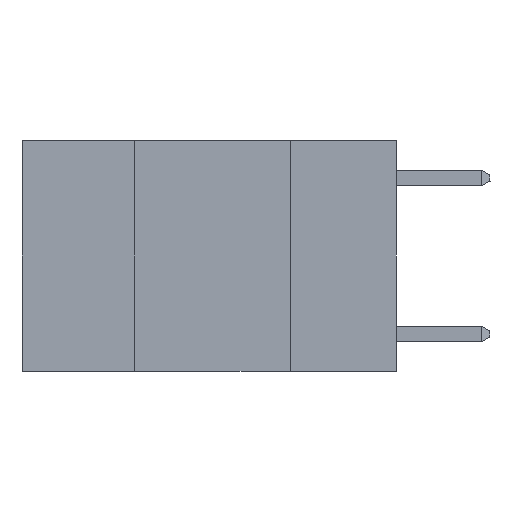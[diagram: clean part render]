
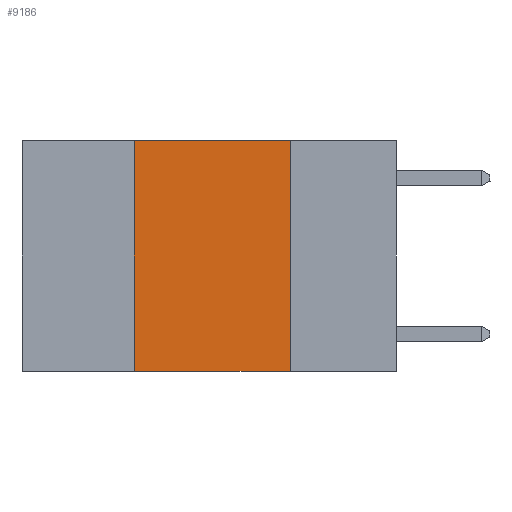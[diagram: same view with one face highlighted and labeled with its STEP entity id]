
A CAD part, left-side view. The second image highlights one B-rep face of the part: STEP entity #9186.
In plain terms, the highlighted planar face has unit normal (-1, 0, 0).
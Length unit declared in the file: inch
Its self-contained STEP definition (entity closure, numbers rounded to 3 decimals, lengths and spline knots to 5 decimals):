
#835 = DIRECTION ( 'NONE',  ( 1., 0., 0. ) ) ;
#1082 = LINE ( 'NONE', #6407, #12794 ) ;
#1088 = EDGE_CURVE ( 'NONE', #3923, #10130, #10971, .T. ) ;
#1261 = ORIENTED_EDGE ( 'NONE', *, *, #7226, .F. ) ;
#1346 = EDGE_LOOP ( 'NONE', ( #1261, #1732, #10259, #10201 ) ) ;
#1732 = ORIENTED_EDGE ( 'NONE', *, *, #13590, .F. ) ;
#1974 = CARTESIAN_POINT ( 'NONE',  ( 0., 0.6, -0.37 ) ) ;
#3923 = VERTEX_POINT ( 'NONE', #12865 ) ;
#4222 = VECTOR ( 'NONE', #9239, 39.37008 ) ;
#4973 = VERTEX_POINT ( 'NONE', #9464 ) ;
#4996 = VERTEX_POINT ( 'NONE', #14791 ) ;
#5089 = CARTESIAN_POINT ( 'NONE',  ( 0., 0.17, -0.37 ) ) ;
#6407 = CARTESIAN_POINT ( 'NONE',  ( 0., 0.42, 0. ) ) ;
#7226 = EDGE_CURVE ( 'NONE', #4996, #10130, #16130, .T. ) ;
#7689 = DIRECTION ( 'NONE',  ( 0., -1., 0. ) ) ;
#7904 = DIRECTION ( 'NONE',  ( 0., 0., 1. ) ) ;
#8359 = VECTOR ( 'NONE', #9865, 39.37008 ) ;
#8375 = CARTESIAN_POINT ( 'NONE',  ( 0., 0.17, 0. ) ) ;
#8758 = AXIS2_PLACEMENT_3D ( 'NONE', #18697, #835, #11570 ) ;
#9186 = ADVANCED_FACE ( 'NONE', ( #17589 ), #14385, .F. ) ;
#9239 = DIRECTION ( 'NONE',  ( 0., -1., 0. ) ) ;
#9464 = CARTESIAN_POINT ( 'NONE',  ( 0., 0.42, 0. ) ) ;
#9865 = DIRECTION ( 'NONE',  ( 0., 0., -1. ) ) ;
#10130 = VERTEX_POINT ( 'NONE', #5089 ) ;
#10201 = ORIENTED_EDGE ( 'NONE', *, *, #1088, .T. ) ;
#10259 = ORIENTED_EDGE ( 'NONE', *, *, #18761, .F. ) ;
#10971 = LINE ( 'NONE', #1974, #18172 ) ;
#11570 = DIRECTION ( 'NONE',  ( 0., 0., -1. ) ) ;
#12220 = CARTESIAN_POINT ( 'NONE',  ( 0., 0.6, 0. ) ) ;
#12274 = LINE ( 'NONE', #12220, #4222 ) ;
#12794 = VECTOR ( 'NONE', #7904, 39.37008 ) ;
#12865 = CARTESIAN_POINT ( 'NONE',  ( 0., 0.42, -0.37 ) ) ;
#13590 = EDGE_CURVE ( 'NONE', #4973, #4996, #12274, .T. ) ;
#14385 = PLANE ( 'NONE',  #8758 ) ;
#14791 = CARTESIAN_POINT ( 'NONE',  ( 0., 0.17, 0. ) ) ;
#16130 = LINE ( 'NONE', #8375, #8359 ) ;
#17589 = FACE_OUTER_BOUND ( 'NONE', #1346, .T. ) ;
#18172 = VECTOR ( 'NONE', #7689, 39.37008 ) ;
#18697 = CARTESIAN_POINT ( 'NONE',  ( 0., 0.6, 0. ) ) ;
#18761 = EDGE_CURVE ( 'NONE', #3923, #4973, #1082, .T. ) ;
